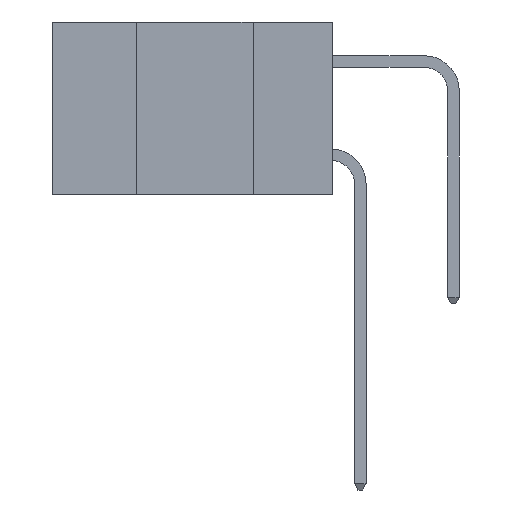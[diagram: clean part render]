
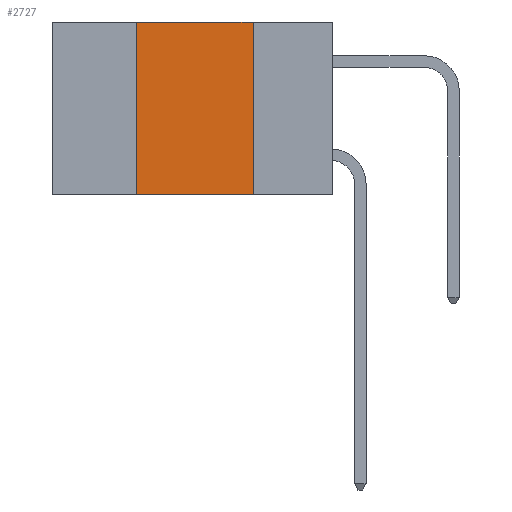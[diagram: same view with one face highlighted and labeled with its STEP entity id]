
A CAD part, left-side view. The second image highlights one B-rep face of the part: STEP entity #2727.
In plain terms, the highlighted planar face has unit normal (-1, 0, 0).
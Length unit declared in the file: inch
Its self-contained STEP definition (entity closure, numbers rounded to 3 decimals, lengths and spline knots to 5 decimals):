
#432 = ORIENTED_EDGE ( 'NONE', *, *, #8632, .F. ) ;
#531 = VERTEX_POINT ( 'NONE', #20922 ) ;
#1084 = EDGE_CURVE ( 'NONE', #7674, #7248, #3073, .T. ) ;
#1511 = EDGE_CURVE ( 'NONE', #9617, #7248, #12331, .T. ) ;
#2279 = LINE ( 'NONE', #19969, #6438 ) ;
#2319 = DIRECTION ( 'NONE',  ( 0., 0., 1. ) ) ;
#2727 = ADVANCED_FACE ( 'NONE', ( #10936 ), #15152, .F. ) ;
#3073 = LINE ( 'NONE', #3282, #15822 ) ;
#3282 = CARTESIAN_POINT ( 'NONE',  ( 0., 0.17, -0.37 ) ) ;
#3440 = CARTESIAN_POINT ( 'NONE',  ( 0., 0.42, -0.37 ) ) ;
#3788 = AXIS2_PLACEMENT_3D ( 'NONE', #15471, #14814, #14812 ) ;
#4008 = ORIENTED_EDGE ( 'NONE', *, *, #1084, .F. ) ;
#5118 = ORIENTED_EDGE ( 'NONE', *, *, #1511, .T. ) ;
#5656 = EDGE_LOOP ( 'NONE', ( #4008, #17794, #432, #5118 ) ) ;
#6134 = DIRECTION ( 'NONE',  ( 0., -1., 0. ) ) ;
#6438 = VECTOR ( 'NONE', #21624, 39.37008 ) ;
#7248 = VERTEX_POINT ( 'NONE', #9155 ) ;
#7674 = VERTEX_POINT ( 'NONE', #20447 ) ;
#7881 = DIRECTION ( 'NONE',  ( 0., 0., -1. ) ) ;
#8632 = EDGE_CURVE ( 'NONE', #9617, #531, #14611, .T. ) ;
#9155 = CARTESIAN_POINT ( 'NONE',  ( 0., 0.17, -0.37 ) ) ;
#9617 = VERTEX_POINT ( 'NONE', #3440 ) ;
#10936 = FACE_OUTER_BOUND ( 'NONE', #5656, .T. ) ;
#11046 = CARTESIAN_POINT ( 'NONE',  ( 0., 0.42, -0.37 ) ) ;
#12331 = LINE ( 'NONE', #19538, #20798 ) ;
#14078 = VECTOR ( 'NONE', #2319, 39.37008 ) ;
#14611 = LINE ( 'NONE', #11046, #14078 ) ;
#14812 = DIRECTION ( 'NONE',  ( 0., 0., -1. ) ) ;
#14814 = DIRECTION ( 'NONE',  ( 1., 0., 0. ) ) ;
#15152 = PLANE ( 'NONE',  #3788 ) ;
#15471 = CARTESIAN_POINT ( 'NONE',  ( 0., 0.6, 0. ) ) ;
#15822 = VECTOR ( 'NONE', #7881, 39.37008 ) ;
#17794 = ORIENTED_EDGE ( 'NONE', *, *, #18914, .F. ) ;
#18914 = EDGE_CURVE ( 'NONE', #531, #7674, #2279, .T. ) ;
#19538 = CARTESIAN_POINT ( 'NONE',  ( 0., 0.6, -0.37 ) ) ;
#19969 = CARTESIAN_POINT ( 'NONE',  ( 0., 0.6, 0. ) ) ;
#20447 = CARTESIAN_POINT ( 'NONE',  ( 0., 0.17, 0. ) ) ;
#20798 = VECTOR ( 'NONE', #6134, 39.37008 ) ;
#20922 = CARTESIAN_POINT ( 'NONE',  ( 0., 0.42, 0. ) ) ;
#21624 = DIRECTION ( 'NONE',  ( 0., -1., 0. ) ) ;
